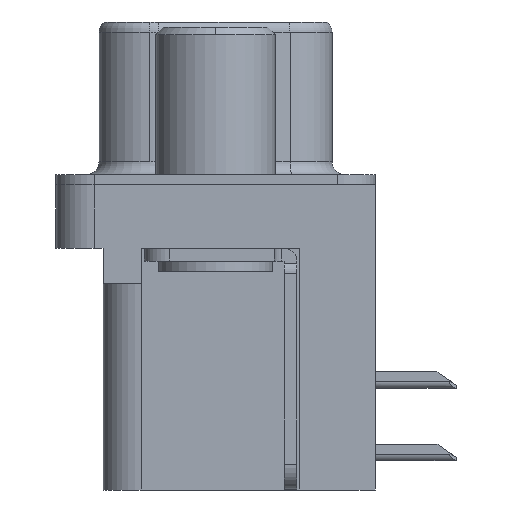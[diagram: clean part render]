
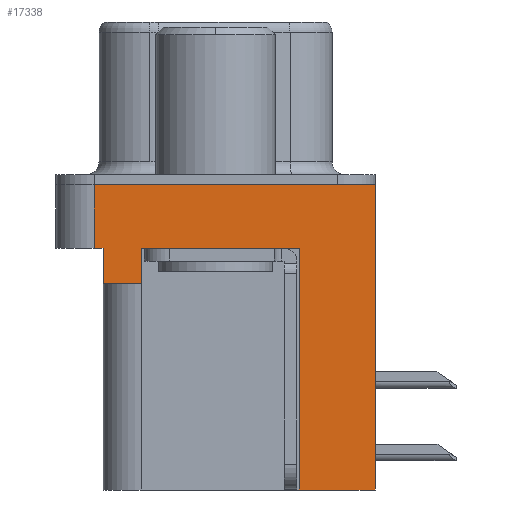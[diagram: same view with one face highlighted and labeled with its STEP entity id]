
A CAD part, left-side view. The second image highlights one B-rep face of the part: STEP entity #17338.
In plain terms, the highlighted planar face has unit normal (-1, 0, 0).
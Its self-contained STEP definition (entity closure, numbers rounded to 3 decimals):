
#634 = VERTEX_POINT ( 'NONE', #15815 ) ;
#718 = CARTESIAN_POINT ( 'NONE',  ( -2.935, 4.425, -3.9 ) ) ;
#1135 = CARTESIAN_POINT ( 'NONE',  ( -2.935, 4.425, -3.9 ) ) ;
#1591 = LINE ( 'NONE', #1135, #3899 ) ;
#2322 = DIRECTION ( 'NONE',  ( 0., 1., 0. ) ) ;
#2502 = EDGE_CURVE ( 'NONE', #634, #13836, #12903, .T. ) ;
#2816 = VECTOR ( 'NONE', #8019, 1000. ) ;
#2898 = CARTESIAN_POINT ( 'NONE',  ( -2.935, 4.775, 0. ) ) ;
#3278 = VERTEX_POINT ( 'NONE', #18166 ) ;
#3383 = EDGE_CURVE ( 'NONE', #10288, #3911, #12629, .T. ) ;
#3523 = LINE ( 'NONE', #16729, #2816 ) ;
#3526 = LINE ( 'NONE', #11722, #16807 ) ;
#3750 = CARTESIAN_POINT ( 'NONE',  ( -2.935, -6.275, -12. ) ) ;
#3899 = VECTOR ( 'NONE', #15766, 1000. ) ;
#3911 = VERTEX_POINT ( 'NONE', #2898 ) ;
#4047 = DIRECTION ( 'NONE',  ( 0., 1., 0. ) ) ;
#4161 = EDGE_CURVE ( 'NONE', #13836, #15044, #1591, .T. ) ;
#4231 = CARTESIAN_POINT ( 'NONE',  ( -2.935, 4.425, -2.5 ) ) ;
#4338 = DIRECTION ( 'NONE',  ( 0., 0., 1. ) ) ;
#4597 = VECTOR ( 'NONE', #4338, 1000. ) ;
#4770 = VERTEX_POINT ( 'NONE', #5398 ) ;
#5046 = VECTOR ( 'NONE', #8009, 1000. ) ;
#5398 = CARTESIAN_POINT ( 'NONE',  ( -2.935, 2.895, -2.5 ) ) ;
#5629 = PLANE ( 'NONE',  #11925 ) ;
#5796 = CARTESIAN_POINT ( 'NONE',  ( -2.935, -6.275, 0. ) ) ;
#5810 = VECTOR ( 'NONE', #15761, 1000. ) ;
#6000 = LINE ( 'NONE', #9982, #14468 ) ;
#6776 = ORIENTED_EDGE ( 'NONE', *, *, #18617, .F. ) ;
#6816 = EDGE_CURVE ( 'NONE', #18476, #3278, #3526, .T. ) ;
#7143 = EDGE_CURVE ( 'NONE', #10288, #15044, #11750, .T. ) ;
#7360 = ORIENTED_EDGE ( 'NONE', *, *, #7143, .T. ) ;
#7405 = ORIENTED_EDGE ( 'NONE', *, *, #10498, .T. ) ;
#7574 = ORIENTED_EDGE ( 'NONE', *, *, #2502, .F. ) ;
#7669 = EDGE_CURVE ( 'NONE', #3911, #12371, #11621, .T. ) ;
#7885 = CARTESIAN_POINT ( 'NONE',  ( -2.935, -6.275, -2.5 ) ) ;
#8009 = DIRECTION ( 'NONE',  ( 0., -1., 0. ) ) ;
#8019 = DIRECTION ( 'NONE',  ( 0., 0., 1. ) ) ;
#8392 = CARTESIAN_POINT ( 'NONE',  ( -2.935, -3.295, -12. ) ) ;
#8516 = VERTEX_POINT ( 'NONE', #3750 ) ;
#9349 = ORIENTED_EDGE ( 'NONE', *, *, #16573, .T. ) ;
#9415 = CARTESIAN_POINT ( 'NONE',  ( -2.935, -3.295, -12. ) ) ;
#9752 = VECTOR ( 'NONE', #4047, 1000. ) ;
#9982 = CARTESIAN_POINT ( 'NONE',  ( -2.935, -6.275, -2.5 ) ) ;
#10021 = VECTOR ( 'NONE', #15987, 1000. ) ;
#10035 = DIRECTION ( 'NONE',  ( 0., 0., 1. ) ) ;
#10288 = VERTEX_POINT ( 'NONE', #15005 ) ;
#10498 = EDGE_CURVE ( 'NONE', #8516, #12371, #6000, .T. ) ;
#10546 = LINE ( 'NONE', #7885, #5046 ) ;
#11448 = CARTESIAN_POINT ( 'NONE',  ( -2.935, 4.775, -2.5 ) ) ;
#11621 = LINE ( 'NONE', #5796, #10021 ) ;
#11722 = CARTESIAN_POINT ( 'NONE',  ( -2.935, -3.295, -12. ) ) ;
#11750 = LINE ( 'NONE', #18640, #5810 ) ;
#11764 = CARTESIAN_POINT ( 'NONE',  ( -2.935, -6.275, -2.5 ) ) ;
#11785 = ORIENTED_EDGE ( 'NONE', *, *, #17763, .T. ) ;
#11925 = AXIS2_PLACEMENT_3D ( 'NONE', #11764, #17353, #10035 ) ;
#12371 = VERTEX_POINT ( 'NONE', #17213 ) ;
#12409 = FACE_OUTER_BOUND ( 'NONE', #16306, .T. ) ;
#12588 = CARTESIAN_POINT ( 'NONE',  ( -2.935, 4.425, -3.9 ) ) ;
#12629 = LINE ( 'NONE', #11448, #4597 ) ;
#12893 = DIRECTION ( 'NONE',  ( 0., 0., 1. ) ) ;
#12903 = LINE ( 'NONE', #718, #17715 ) ;
#12982 = ORIENTED_EDGE ( 'NONE', *, *, #7669, .F. ) ;
#13390 = DIRECTION ( 'NONE',  ( 0., 0., 1. ) ) ;
#13836 = VERTEX_POINT ( 'NONE', #12588 ) ;
#14468 = VECTOR ( 'NONE', #12893, 1000. ) ;
#15005 = CARTESIAN_POINT ( 'NONE',  ( -2.935, 4.775, -2.5 ) ) ;
#15044 = VERTEX_POINT ( 'NONE', #4231 ) ;
#15761 = DIRECTION ( 'NONE',  ( 0., -1., 0. ) ) ;
#15766 = DIRECTION ( 'NONE',  ( 0., 0., 1. ) ) ;
#15815 = CARTESIAN_POINT ( 'NONE',  ( -2.935, 2.895, -3.9 ) ) ;
#15987 = DIRECTION ( 'NONE',  ( 0., -1., 0. ) ) ;
#16306 = EDGE_LOOP ( 'NONE', ( #12982, #17088, #7360, #17156, #7574, #9349, #11785, #16439, #6776, #7405 ) ) ;
#16439 = ORIENTED_EDGE ( 'NONE', *, *, #6816, .F. ) ;
#16573 = EDGE_CURVE ( 'NONE', #634, #4770, #3523, .T. ) ;
#16729 = CARTESIAN_POINT ( 'NONE',  ( -2.935, 2.895, -3.9 ) ) ;
#16807 = VECTOR ( 'NONE', #13390, 1000. ) ;
#17088 = ORIENTED_EDGE ( 'NONE', *, *, #3383, .F. ) ;
#17156 = ORIENTED_EDGE ( 'NONE', *, *, #4161, .F. ) ;
#17213 = CARTESIAN_POINT ( 'NONE',  ( -2.935, -6.275, 0. ) ) ;
#17338 = ADVANCED_FACE ( 'NONE', ( #12409 ), #5629, .T. ) ;
#17353 = DIRECTION ( 'NONE',  ( -1., 0., 0. ) ) ;
#17715 = VECTOR ( 'NONE', #2322, 1000. ) ;
#17763 = EDGE_CURVE ( 'NONE', #4770, #3278, #10546, .T. ) ;
#18166 = CARTESIAN_POINT ( 'NONE',  ( -2.935, -3.295, -2.5 ) ) ;
#18271 = LINE ( 'NONE', #8392, #9752 ) ;
#18476 = VERTEX_POINT ( 'NONE', #9415 ) ;
#18617 = EDGE_CURVE ( 'NONE', #8516, #18476, #18271, .T. ) ;
#18640 = CARTESIAN_POINT ( 'NONE',  ( -2.935, -6.275, -2.5 ) ) ;
